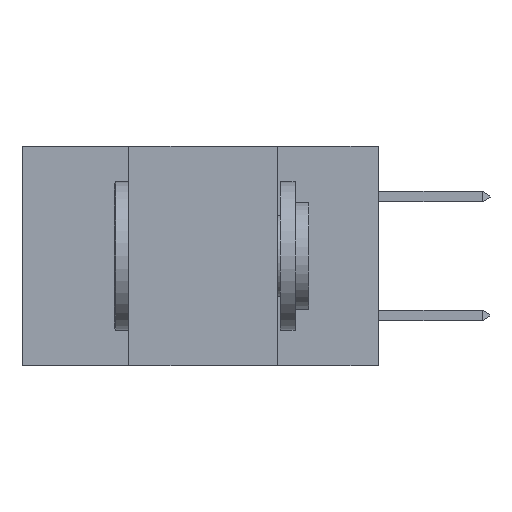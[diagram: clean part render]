
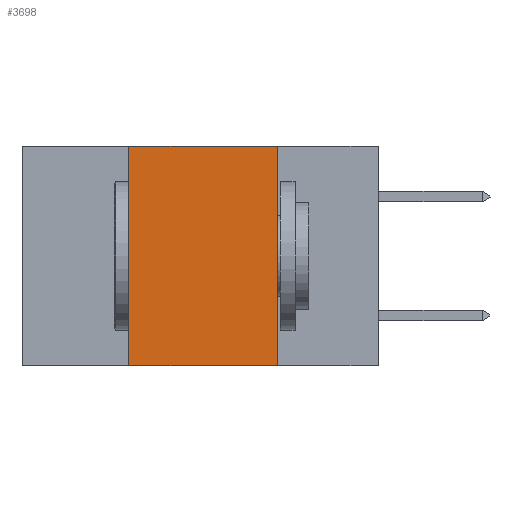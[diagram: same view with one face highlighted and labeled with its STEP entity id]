
A CAD part, left-side view. The second image highlights one B-rep face of the part: STEP entity #3698.
In plain terms, the highlighted planar face has unit normal (-1, 0, 0).
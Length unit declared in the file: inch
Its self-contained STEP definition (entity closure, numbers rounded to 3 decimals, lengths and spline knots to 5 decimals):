
#528 = CARTESIAN_POINT ( 'NONE',  ( 0., 0.42, -0.37 ) ) ;
#885 = CARTESIAN_POINT ( 'NONE',  ( 0., 0.17, 0. ) ) ;
#1101 = FACE_OUTER_BOUND ( 'NONE', #22220, .T. ) ;
#1460 = DIRECTION ( 'NONE',  ( 0., -1., 0. ) ) ;
#3414 = ORIENTED_EDGE ( 'NONE', *, *, #14505, .F. ) ;
#3698 = ADVANCED_FACE ( 'NONE', ( #1101 ), #15600, .F. ) ;
#4638 = CARTESIAN_POINT ( 'NONE',  ( 0., 0.17, -0.37 ) ) ;
#5006 = VERTEX_POINT ( 'NONE', #10556 ) ;
#6372 = LINE ( 'NONE', #24667, #12415 ) ;
#8674 = EDGE_CURVE ( 'NONE', #17316, #10411, #6372, .T. ) ;
#8944 = EDGE_CURVE ( 'NONE', #5006, #12378, #20619, .T. ) ;
#10154 = DIRECTION ( 'NONE',  ( 0., 0., -1. ) ) ;
#10211 = DIRECTION ( 'NONE',  ( 0., -1., 0. ) ) ;
#10411 = VERTEX_POINT ( 'NONE', #4638 ) ;
#10556 = CARTESIAN_POINT ( 'NONE',  ( 0., 0.42, 0. ) ) ;
#11763 = CARTESIAN_POINT ( 'NONE',  ( 0., 0.6, 0. ) ) ;
#12378 = VERTEX_POINT ( 'NONE', #14209 ) ;
#12415 = VECTOR ( 'NONE', #1460, 39.37008 ) ;
#12556 = VECTOR ( 'NONE', #17948, 39.37008 ) ;
#14209 = CARTESIAN_POINT ( 'NONE',  ( 0., 0.17, 0. ) ) ;
#14505 = EDGE_CURVE ( 'NONE', #12378, #10411, #16939, .T. ) ;
#15544 = AXIS2_PLACEMENT_3D ( 'NONE', #11763, #21741, #10154 ) ;
#15600 = PLANE ( 'NONE',  #15544 ) ;
#15827 = CARTESIAN_POINT ( 'NONE',  ( 0., 0.6, 0. ) ) ;
#16199 = LINE ( 'NONE', #21977, #12556 ) ;
#16939 = LINE ( 'NONE', #885, #20264 ) ;
#17316 = VERTEX_POINT ( 'NONE', #528 ) ;
#17948 = DIRECTION ( 'NONE',  ( 0., 0., 1. ) ) ;
#20227 = DIRECTION ( 'NONE',  ( 0., 0., -1. ) ) ;
#20264 = VECTOR ( 'NONE', #20227, 39.37008 ) ;
#20619 = LINE ( 'NONE', #15827, #23016 ) ;
#21741 = DIRECTION ( 'NONE',  ( 1., 0., 0. ) ) ;
#21854 = ORIENTED_EDGE ( 'NONE', *, *, #8944, .F. ) ;
#21977 = CARTESIAN_POINT ( 'NONE',  ( 0., 0.42, 0. ) ) ;
#22220 = EDGE_LOOP ( 'NONE', ( #3414, #21854, #24726, #23778 ) ) ;
#22439 = EDGE_CURVE ( 'NONE', #17316, #5006, #16199, .T. ) ;
#23016 = VECTOR ( 'NONE', #10211, 39.37008 ) ;
#23778 = ORIENTED_EDGE ( 'NONE', *, *, #8674, .T. ) ;
#24667 = CARTESIAN_POINT ( 'NONE',  ( 0., 0.6, -0.37 ) ) ;
#24726 = ORIENTED_EDGE ( 'NONE', *, *, #22439, .F. ) ;
